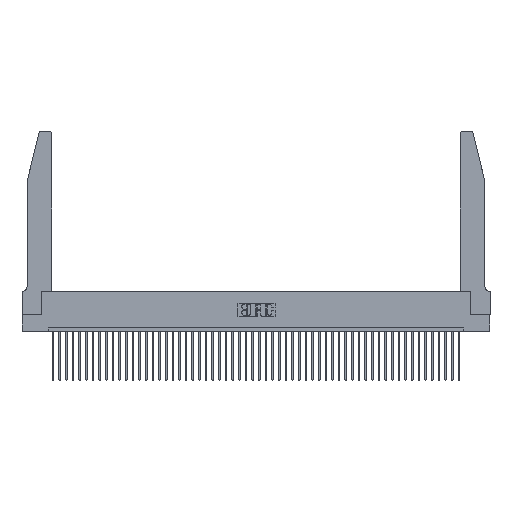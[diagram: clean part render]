
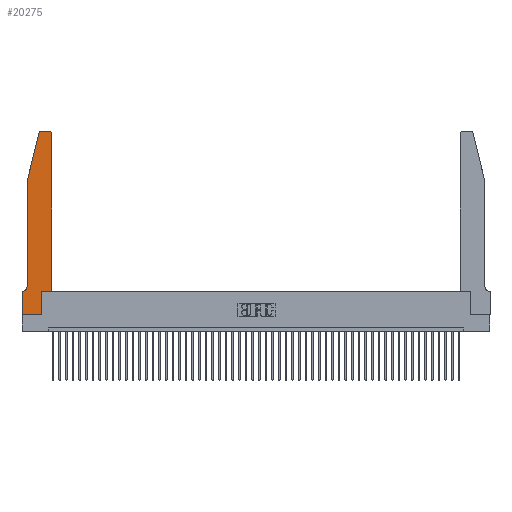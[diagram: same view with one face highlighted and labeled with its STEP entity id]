
A CAD part, top view. The second image highlights one B-rep face of the part: STEP entity #20275.
In plain terms, the highlighted planar face has unit normal (0, 0, 1).
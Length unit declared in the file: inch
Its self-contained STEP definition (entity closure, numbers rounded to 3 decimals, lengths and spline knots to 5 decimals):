
#421 = ORIENTED_EDGE ( 'NONE', *, *, #21036, .T. ) ;
#494 = AXIS2_PLACEMENT_3D ( 'NONE', #26980, #23364, #8349 ) ;
#1230 = EDGE_CURVE ( 'NONE', #5917, #20623, #17473, .T. ) ;
#1431 = VECTOR ( 'NONE', #25541, 39.37008 ) ;
#1946 = CARTESIAN_POINT ( 'NONE',  ( 0., 0., 0.37 ) ) ;
#2054 = EDGE_CURVE ( 'NONE', #10245, #4617, #32695, .T. ) ;
#2646 = CARTESIAN_POINT ( 'NONE',  ( 0.2865, 0.35, 0.37 ) ) ;
#2764 = VERTEX_POINT ( 'NONE', #10470 ) ;
#4020 = DIRECTION ( 'NONE',  ( 0., 0., 1. ) ) ;
#4162 = DIRECTION ( 'NONE',  ( 0., 0., -1. ) ) ;
#4615 = VECTOR ( 'NONE', #24604, 39.37008 ) ;
#4617 = VERTEX_POINT ( 'NONE', #41416 ) ;
#4637 = DIRECTION ( 'NONE',  ( 0., 1., 0. ) ) ;
#5826 = EDGE_CURVE ( 'NONE', #14836, #5845, #8158, .T. ) ;
#5845 = VERTEX_POINT ( 'NONE', #8763 ) ;
#5917 = VERTEX_POINT ( 'NONE', #8930 ) ;
#6225 = CARTESIAN_POINT ( 'NONE',  ( 0.25487, 2.72718, 0.37 ) ) ;
#7029 = VERTEX_POINT ( 'NONE', #2646 ) ;
#8158 = LINE ( 'NONE', #46036, #4615 ) ;
#8349 = DIRECTION ( 'NONE',  ( 1., 0., 0. ) ) ;
#8763 = CARTESIAN_POINT ( 'NONE',  ( 0.2865, 0., 0.37 ) ) ;
#8930 = CARTESIAN_POINT ( 'NONE',  ( 0.284, 2.75, 0.37 ) ) ;
#8962 = ORIENTED_EDGE ( 'NONE', *, *, #1230, .T. ) ;
#9011 = VERTEX_POINT ( 'NONE', #15090 ) ;
#9048 = VERTEX_POINT ( 'NONE', #28541 ) ;
#9111 = AXIS2_PLACEMENT_3D ( 'NONE', #34595, #4162, #19947 ) ;
#9461 = CARTESIAN_POINT ( 'NONE',  ( 0.2865, 0.35, 0.37 ) ) ;
#9822 = VECTOR ( 'NONE', #21859, 39.37008 ) ;
#10245 = VERTEX_POINT ( 'NONE', #20785 ) ;
#10361 = CARTESIAN_POINT ( 'NONE',  ( 0.4505, 0.35, 0.37 ) ) ;
#10470 = CARTESIAN_POINT ( 'NONE',  ( 0.0755, 0.42, 0.37 ) ) ;
#11010 = VECTOR ( 'NONE', #41551, 39.37008 ) ;
#11328 = DIRECTION ( 'NONE',  ( -1., 0., 0. ) ) ;
#11368 = CARTESIAN_POINT ( 'NONE',  ( 0.2605, 2.75, 0.37 ) ) ;
#12734 = VECTOR ( 'NONE', #31098, 39.37008 ) ;
#13574 = VERTEX_POINT ( 'NONE', #39037 ) ;
#14836 = VERTEX_POINT ( 'NONE', #1946 ) ;
#15061 = AXIS2_PLACEMENT_3D ( 'NONE', #19203, #34203, #19521 ) ;
#15090 = CARTESIAN_POINT ( 'NONE',  ( 0.4205, 2.75, 0.37 ) ) ;
#15587 = LINE ( 'NONE', #10361, #1431 ) ;
#16981 = CARTESIAN_POINT ( 'NONE',  ( 0.0755, 2., 0.37 ) ) ;
#16983 = ORIENTED_EDGE ( 'NONE', *, *, #27122, .T. ) ;
#17473 = CIRCLE ( 'NONE', #15061, 0.03 ) ;
#18221 = ORIENTED_EDGE ( 'NONE', *, *, #5826, .T. ) ;
#18758 = ORIENTED_EDGE ( 'NONE', *, *, #38460, .T. ) ;
#19203 = CARTESIAN_POINT ( 'NONE',  ( 0.284, 2.72, 0.37 ) ) ;
#19521 = DIRECTION ( 'NONE',  ( 1., 0., 0. ) ) ;
#19947 = DIRECTION ( 'NONE',  ( -1., 0., 0. ) ) ;
#20117 = VECTOR ( 'NONE', #4637, 39.37008 ) ;
#20141 = EDGE_CURVE ( 'NONE', #4617, #9011, #29272, .T. ) ;
#20275 = ADVANCED_FACE ( 'NONE', ( #41672 ), #25747, .T. ) ;
#20623 = VERTEX_POINT ( 'NONE', #6225 ) ;
#20785 = CARTESIAN_POINT ( 'NONE',  ( 0.4505, 0.35, 0.37 ) ) ;
#21036 = EDGE_CURVE ( 'NONE', #9011, #5917, #41461, .T. ) ;
#21518 = EDGE_CURVE ( 'NONE', #28076, #13574, #33708, .T. ) ;
#21859 = DIRECTION ( 'NONE',  ( 0., -1., 0. ) ) ;
#22715 = VECTOR ( 'NONE', #40870, 39.37008 ) ;
#22737 = CARTESIAN_POINT ( 'NONE',  ( 0.0755, 2., 0.37 ) ) ;
#23364 = DIRECTION ( 'NONE',  ( 0., 0., 1. ) ) ;
#23660 = LINE ( 'NONE', #9461, #20117 ) ;
#24229 = EDGE_CURVE ( 'NONE', #13574, #14836, #38139, .T. ) ;
#24574 = ORIENTED_EDGE ( 'NONE', *, *, #44964, .T. ) ;
#24604 = DIRECTION ( 'NONE',  ( 1., 0., 0. ) ) ;
#25314 = CIRCLE ( 'NONE', #9111, 0.07 ) ;
#25346 = EDGE_CURVE ( 'NONE', #7029, #10245, #15587, .T. ) ;
#25541 = DIRECTION ( 'NONE',  ( 1., 0., 0. ) ) ;
#25747 = PLANE ( 'NONE',  #494 ) ;
#26980 = CARTESIAN_POINT ( 'NONE',  ( 0., 0.35, 0.37 ) ) ;
#27122 = EDGE_CURVE ( 'NONE', #9048, #2764, #36365, .T. ) ;
#28076 = VERTEX_POINT ( 'NONE', #31434 ) ;
#28541 = CARTESIAN_POINT ( 'NONE',  ( 0.0755, 2., 0.37 ) ) ;
#28801 = ORIENTED_EDGE ( 'NONE', *, *, #25346, .T. ) ;
#29272 = CIRCLE ( 'NONE', #41880, 0.03 ) ;
#29597 = ORIENTED_EDGE ( 'NONE', *, *, #20141, .T. ) ;
#31098 = DIRECTION ( 'NONE',  ( 0., -1., 0. ) ) ;
#31336 = ORIENTED_EDGE ( 'NONE', *, *, #21518, .T. ) ;
#31434 = CARTESIAN_POINT ( 'NONE',  ( 0.0055, 0.35, 0.37 ) ) ;
#32695 = LINE ( 'NONE', #44632, #22715 ) ;
#33662 = EDGE_CURVE ( 'NONE', #2764, #28076, #25314, .T. ) ;
#33708 = LINE ( 'NONE', #45904, #40801 ) ;
#33992 = CARTESIAN_POINT ( 'NONE',  ( 0.4205, 2.72, 0.37 ) ) ;
#34203 = DIRECTION ( 'NONE',  ( 0., 0., 1. ) ) ;
#34595 = CARTESIAN_POINT ( 'NONE',  ( 0.0055, 0.42, 0.37 ) ) ;
#36365 = LINE ( 'NONE', #16981, #12734 ) ;
#37365 = VECTOR ( 'NONE', #38066, 39.37008 ) ;
#37993 = DIRECTION ( 'NONE',  ( 1., 0., 0. ) ) ;
#38066 = DIRECTION ( 'NONE',  ( -1., 0., 0. ) ) ;
#38139 = LINE ( 'NONE', #48215, #9822 ) ;
#38460 = EDGE_CURVE ( 'NONE', #5845, #7029, #23660, .T. ) ;
#39037 = CARTESIAN_POINT ( 'NONE',  ( 0., 0.35, 0.37 ) ) ;
#39492 = ORIENTED_EDGE ( 'NONE', *, *, #33662, .T. ) ;
#40801 = VECTOR ( 'NONE', #11328, 39.37008 ) ;
#40870 = DIRECTION ( 'NONE',  ( 0., 1., 0. ) ) ;
#41416 = CARTESIAN_POINT ( 'NONE',  ( 0.4505, 2.72, 0.37 ) ) ;
#41428 = ORIENTED_EDGE ( 'NONE', *, *, #2054, .T. ) ;
#41461 = LINE ( 'NONE', #11368, #37365 ) ;
#41551 = DIRECTION ( 'NONE',  ( -0.239, -0.971, 0. ) ) ;
#41672 = FACE_OUTER_BOUND ( 'NONE', #46319, .T. ) ;
#41880 = AXIS2_PLACEMENT_3D ( 'NONE', #33992, #4020, #37993 ) ;
#44632 = CARTESIAN_POINT ( 'NONE',  ( 0.4505, 0.35, 0.37 ) ) ;
#44964 = EDGE_CURVE ( 'NONE', #20623, #9048, #46340, .T. ) ;
#45904 = CARTESIAN_POINT ( 'NONE',  ( 0.0755, 0.35, 0.37 ) ) ;
#46036 = CARTESIAN_POINT ( 'NONE',  ( 0., 0., 0.37 ) ) ;
#46319 = EDGE_LOOP ( 'NONE', ( #421, #8962, #24574, #16983, #39492, #31336, #47711, #18221, #18758, #28801, #41428, #29597 ) ) ;
#46340 = LINE ( 'NONE', #22737, #11010 ) ;
#47711 = ORIENTED_EDGE ( 'NONE', *, *, #24229, .T. ) ;
#48215 = CARTESIAN_POINT ( 'NONE',  ( 0., 0., 0.37 ) ) ;
